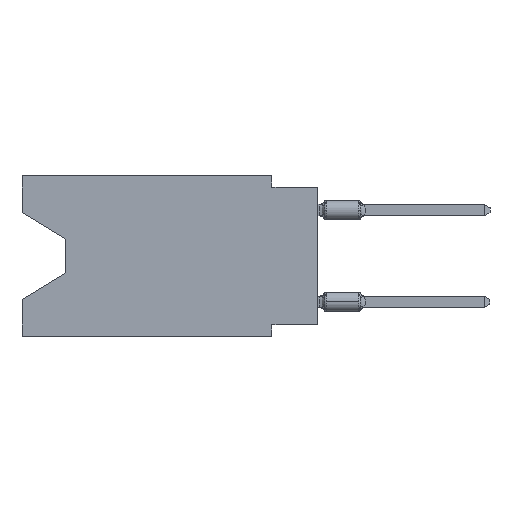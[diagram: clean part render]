
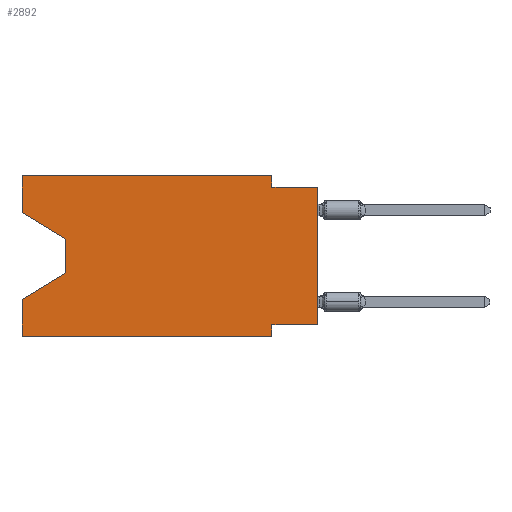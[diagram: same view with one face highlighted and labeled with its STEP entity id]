
A CAD part, left-side view. The second image highlights one B-rep face of the part: STEP entity #2892.
In plain terms, the highlighted planar face has unit normal (-1, 0, 0).
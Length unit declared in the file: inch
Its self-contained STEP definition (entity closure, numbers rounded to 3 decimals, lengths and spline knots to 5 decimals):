
#33 = VERTEX_POINT ( 'NONE', #22226 ) ;
#129 = VECTOR ( 'NONE', #32407, 39.37008 ) ;
#255 = CARTESIAN_POINT ( 'NONE',  ( 0., 0.55, -0.138 ) ) ;
#1011 = ORIENTED_EDGE ( 'NONE', *, *, #1073, .T. ) ;
#1073 = EDGE_CURVE ( 'NONE', #15109, #27737, #12579, .T. ) ;
#1398 = CARTESIAN_POINT ( 'NONE',  ( 0., 0.55, -0.138 ) ) ;
#2451 = DIRECTION ( 'NONE',  ( 0., 0., -1. ) ) ;
#2674 = LINE ( 'NONE', #12434, #14034 ) ;
#2846 = DIRECTION ( 'NONE',  ( 0., 0., 1. ) ) ;
#2892 = ADVANCED_FACE ( 'NONE', ( #22070 ), #14984, .F. ) ;
#3433 = LINE ( 'NONE', #27996, #12041 ) ;
#4390 = ORIENTED_EDGE ( 'NONE', *, *, #16145, .F. ) ;
#4437 = CARTESIAN_POINT ( 'NONE',  ( 0., 0., -0.325 ) ) ;
#4467 = VERTEX_POINT ( 'NONE', #4437 ) ;
#4676 = DIRECTION ( 'NONE',  ( 0., 0.855, -0.519 ) ) ;
#4878 = EDGE_LOOP ( 'NONE', ( #26053, #18973, #1011, #4390, #8132, #10208, #27645, #26619, #17552, #14886, #17074, #14807 ) ) ;
#5530 = DIRECTION ( 'NONE',  ( 0., -1., 0. ) ) ;
#5667 = EDGE_CURVE ( 'NONE', #17179, #17768, #31906, .T. ) ;
#5801 = LINE ( 'NONE', #22960, #25522 ) ;
#5912 = DIRECTION ( 'NONE',  ( 0., 0., 1. ) ) ;
#5935 = EDGE_CURVE ( 'NONE', #4467, #17179, #5801, .T. ) ;
#6093 = LINE ( 'NONE', #12584, #16389 ) ;
#6339 = CARTESIAN_POINT ( 'NONE',  ( 0., 0.1, 0. ) ) ;
#6973 = VERTEX_POINT ( 'NONE', #1398 ) ;
#7837 = EDGE_CURVE ( 'NONE', #33, #8341, #2674, .T. ) ;
#8132 = ORIENTED_EDGE ( 'NONE', *, *, #29494, .T. ) ;
#8341 = VERTEX_POINT ( 'NONE', #22066 ) ;
#9231 = DIRECTION ( 'NONE',  ( 0., -1., 0. ) ) ;
#9347 = EDGE_CURVE ( 'NONE', #6973, #15109, #13099, .T. ) ;
#9879 = DIRECTION ( 'NONE',  ( 0., -0.855, -0.519 ) ) ;
#10083 = CARTESIAN_POINT ( 'NONE',  ( 0., 0.645, -0.26975 ) ) ;
#10208 = ORIENTED_EDGE ( 'NONE', *, *, #5667, .F. ) ;
#10425 = VECTOR ( 'NONE', #25462, 39.37008 ) ;
#11024 = CARTESIAN_POINT ( 'NONE',  ( 0., 0.645, -0.35 ) ) ;
#12041 = VECTOR ( 'NONE', #5912, 39.37008 ) ;
#12434 = CARTESIAN_POINT ( 'NONE',  ( 0., 0.645, 0. ) ) ;
#12517 = CARTESIAN_POINT ( 'NONE',  ( 0., 0.645, 0. ) ) ;
#12579 = LINE ( 'NONE', #30214, #26584 ) ;
#12584 = CARTESIAN_POINT ( 'NONE',  ( 0., 0.645, 0. ) ) ;
#12747 = DIRECTION ( 'NONE',  ( 0., -1., 0. ) ) ;
#13099 = LINE ( 'NONE', #255, #10425 ) ;
#13224 = DIRECTION ( 'NONE',  ( 0., 1., 0. ) ) ;
#14034 = VECTOR ( 'NONE', #12747, 39.37008 ) ;
#14807 = ORIENTED_EDGE ( 'NONE', *, *, #23306, .F. ) ;
#14886 = ORIENTED_EDGE ( 'NONE', *, *, #29833, .F. ) ;
#14984 = PLANE ( 'NONE',  #28616 ) ;
#15109 = VERTEX_POINT ( 'NONE', #25615 ) ;
#15898 = DIRECTION ( 'NONE',  ( 0., 0., -1. ) ) ;
#16051 = EDGE_CURVE ( 'NONE', #16663, #6973, #17475, .T. ) ;
#16145 = EDGE_CURVE ( 'NONE', #20330, #27737, #3433, .T. ) ;
#16389 = VECTOR ( 'NONE', #2846, 39.37008 ) ;
#16413 = CARTESIAN_POINT ( 'NONE',  ( 0., 0.645, -0.08025 ) ) ;
#16663 = VERTEX_POINT ( 'NONE', #16413 ) ;
#16722 = DIRECTION ( 'NONE',  ( 0., 0., -1. ) ) ;
#17074 = ORIENTED_EDGE ( 'NONE', *, *, #7837, .F. ) ;
#17179 = VERTEX_POINT ( 'NONE', #17864 ) ;
#17287 = CARTESIAN_POINT ( 'NONE',  ( 0., 0.1, -0.025 ) ) ;
#17475 = LINE ( 'NONE', #18645, #29404 ) ;
#17552 = ORIENTED_EDGE ( 'NONE', *, *, #26423, .F. ) ;
#17768 = VERTEX_POINT ( 'NONE', #30995 ) ;
#17864 = CARTESIAN_POINT ( 'NONE',  ( 0., 0.1, -0.325 ) ) ;
#18645 = CARTESIAN_POINT ( 'NONE',  ( 0., 0.645, -0.08025 ) ) ;
#18973 = ORIENTED_EDGE ( 'NONE', *, *, #9347, .T. ) ;
#20177 = CARTESIAN_POINT ( 'NONE',  ( 0., 0., 0. ) ) ;
#20330 = VERTEX_POINT ( 'NONE', #23869 ) ;
#20524 = LINE ( 'NONE', #30909, #21718 ) ;
#21718 = VECTOR ( 'NONE', #5530, 39.37008 ) ;
#22066 = CARTESIAN_POINT ( 'NONE',  ( 0., 0.1, 0. ) ) ;
#22070 = FACE_OUTER_BOUND ( 'NONE', #4878, .T. ) ;
#22226 = CARTESIAN_POINT ( 'NONE',  ( 0., 0.645, 0. ) ) ;
#22330 = LINE ( 'NONE', #20177, #129 ) ;
#22960 = CARTESIAN_POINT ( 'NONE',  ( 0., 0., -0.325 ) ) ;
#23306 = EDGE_CURVE ( 'NONE', #16663, #33, #6093, .T. ) ;
#23869 = CARTESIAN_POINT ( 'NONE',  ( 0., 0.645, -0.35 ) ) ;
#23894 = VERTEX_POINT ( 'NONE', #28914 ) ;
#25462 = DIRECTION ( 'NONE',  ( 0., 0., -1. ) ) ;
#25522 = VECTOR ( 'NONE', #13224, 39.37008 ) ;
#25615 = CARTESIAN_POINT ( 'NONE',  ( 0., 0.55, -0.212 ) ) ;
#25690 = VERTEX_POINT ( 'NONE', #17287 ) ;
#26044 = LINE ( 'NONE', #11024, #31618 ) ;
#26053 = ORIENTED_EDGE ( 'NONE', *, *, #16051, .T. ) ;
#26423 = EDGE_CURVE ( 'NONE', #25690, #23894, #20524, .T. ) ;
#26584 = VECTOR ( 'NONE', #4676, 39.37008 ) ;
#26619 = ORIENTED_EDGE ( 'NONE', *, *, #26774, .T. ) ;
#26774 = EDGE_CURVE ( 'NONE', #4467, #23894, #22330, .T. ) ;
#27645 = ORIENTED_EDGE ( 'NONE', *, *, #5935, .F. ) ;
#27737 = VERTEX_POINT ( 'NONE', #10083 ) ;
#27996 = CARTESIAN_POINT ( 'NONE',  ( 0., 0.645, 0. ) ) ;
#28616 = AXIS2_PLACEMENT_3D ( 'NONE', #12517, #32481, #2451 ) ;
#28914 = CARTESIAN_POINT ( 'NONE',  ( 0., 0., -0.025 ) ) ;
#29404 = VECTOR ( 'NONE', #9879, 39.37008 ) ;
#29494 = EDGE_CURVE ( 'NONE', #20330, #17768, #26044, .T. ) ;
#29732 = VECTOR ( 'NONE', #16722, 39.37008 ) ;
#29833 = EDGE_CURVE ( 'NONE', #8341, #25690, #31408, .T. ) ;
#30214 = CARTESIAN_POINT ( 'NONE',  ( 0., 0.55, -0.212 ) ) ;
#30551 = VECTOR ( 'NONE', #15898, 39.37008 ) ;
#30909 = CARTESIAN_POINT ( 'NONE',  ( 0., 0., -0.025 ) ) ;
#30995 = CARTESIAN_POINT ( 'NONE',  ( 0., 0.1, -0.35 ) ) ;
#31399 = CARTESIAN_POINT ( 'NONE',  ( 0., 0.1, -0.35 ) ) ;
#31408 = LINE ( 'NONE', #6339, #30551 ) ;
#31618 = VECTOR ( 'NONE', #9231, 39.37008 ) ;
#31906 = LINE ( 'NONE', #31399, #29732 ) ;
#32407 = DIRECTION ( 'NONE',  ( 0., 0., 1. ) ) ;
#32481 = DIRECTION ( 'NONE',  ( 1., 0., 0. ) ) ;
